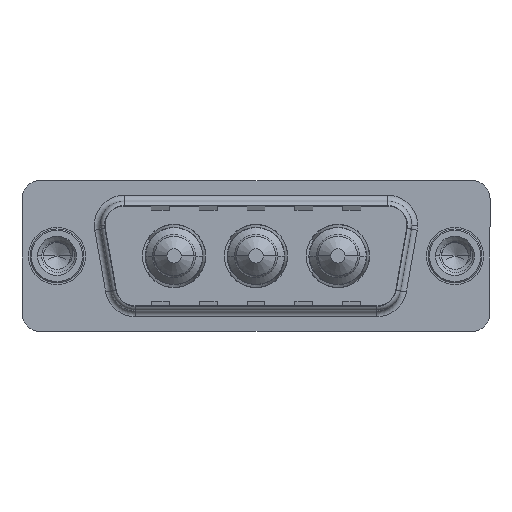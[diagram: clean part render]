
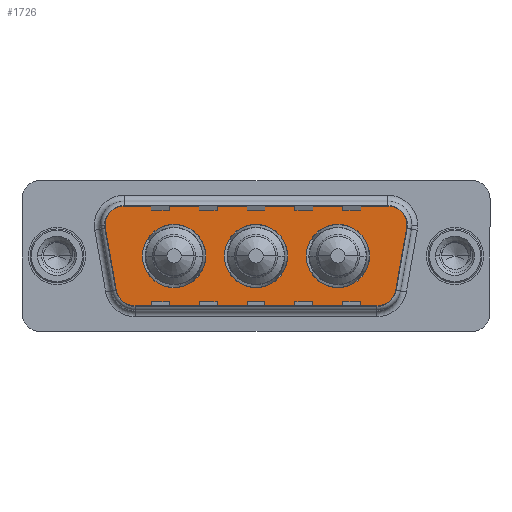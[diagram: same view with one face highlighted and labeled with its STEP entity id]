
A CAD part, top view. The second image highlights one B-rep face of the part: STEP entity #1726.
In plain terms, the highlighted planar face has unit normal (0, 0, 1).
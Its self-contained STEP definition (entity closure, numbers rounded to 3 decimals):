
#42 = DIRECTION ( 'NONE',  ( -1., 0., 0. ) ) ;
#144 = ORIENTED_EDGE ( 'NONE', *, *, #1519, .T. ) ;
#194 = VERTEX_POINT ( 'NONE', #1697 ) ;
#228 = ORIENTED_EDGE ( 'NONE', *, *, #12312, .T. ) ;
#421 = DIRECTION ( 'NONE',  ( 1., 0., 0. ) ) ;
#570 = CIRCLE ( 'NONE', #4856, 2.65 ) ;
#596 = EDGE_CURVE ( 'NONE', #746, #11127, #5800, .T. ) ;
#746 = VERTEX_POINT ( 'NONE', #1865 ) ;
#846 = VERTEX_POINT ( 'NONE', #6445 ) ;
#915 = EDGE_CURVE ( 'NONE', #5797, #9827, #9439, .T. ) ;
#993 = DIRECTION ( 'NONE',  ( 1., 0., 0. ) ) ;
#1413 = AXIS2_PLACEMENT_3D ( 'NONE', #8962, #9779, #2746 ) ;
#1519 = EDGE_CURVE ( 'NONE', #9827, #6201, #9106, .T. ) ;
#1533 = ORIENTED_EDGE ( 'NONE', *, *, #2544, .T. ) ;
#1560 = EDGE_CURVE ( 'NONE', #12996, #7436, #6411, .T. ) ;
#1632 = AXIS2_PLACEMENT_3D ( 'NONE', #11360, #8532, #8520 ) ;
#1697 = CARTESIAN_POINT ( 'NONE',  ( 3.441, 2.553, 0. ) ) ;
#1726 = ADVANCED_FACE ( 'NONE', ( #7830, #2380, #12896, #13206 ), #9777, .T. ) ;
#1814 = DIRECTION ( 'NONE',  ( 0.174, 0.985, 0. ) ) ;
#1865 = CARTESIAN_POINT ( 'NONE',  ( 7.15, 0., 0. ) ) ;
#2040 = VECTOR ( 'NONE', #5356, 1000. ) ;
#2229 = AXIS2_PLACEMENT_3D ( 'NONE', #11794, #5753, #12817 ) ;
#2326 = DIRECTION ( 'NONE',  ( 0., 0., 1. ) ) ;
#2380 = FACE_BOUND ( 'NONE', #3631, .T. ) ;
#2398 = CIRCLE ( 'NONE', #2229, 2.65 ) ;
#2465 = EDGE_CURVE ( 'NONE', #9430, #2941, #10359, .T. ) ;
#2533 = DIRECTION ( 'NONE',  ( -1., 0., 0. ) ) ;
#2544 = EDGE_CURVE ( 'NONE', #194, #12849, #7321, .T. ) ;
#2681 = AXIS2_PLACEMENT_3D ( 'NONE', #4132, #11233, #5159 ) ;
#2745 = ORIENTED_EDGE ( 'NONE', *, *, #2465, .F. ) ;
#2746 = DIRECTION ( 'NONE',  ( 1., 0., 0. ) ) ;
#2854 = ORIENTED_EDGE ( 'NONE', *, *, #5192, .F. ) ;
#2876 = CARTESIAN_POINT ( 'NONE',  ( 6.434, -2.9, 0. ) ) ;
#2888 = CARTESIAN_POINT ( 'NONE',  ( 4.464, -3.247, 0. ) ) ;
#2941 = VERTEX_POINT ( 'NONE', #13060 ) ;
#2987 = ORIENTED_EDGE ( 'NONE', *, *, #1560, .T. ) ;
#3088 = AXIS2_PLACEMENT_3D ( 'NONE', #11510, #12285, #421 ) ;
#3631 = EDGE_LOOP ( 'NONE', ( #2745, #2854 ) ) ;
#3735 = ORIENTED_EDGE ( 'NONE', *, *, #596, .F. ) ;
#3815 = CARTESIAN_POINT ( 'NONE',  ( 5.411, 4.9, 0. ) ) ;
#3872 = LINE ( 'NONE', #3815, #11345 ) ;
#3898 = DIRECTION ( 'NONE',  ( -1., 0., 0. ) ) ;
#3949 = CIRCLE ( 'NONE', #6325, 2. ) ;
#4007 = CARTESIAN_POINT ( 'NONE',  ( 27.889, 2.9, 0. ) ) ;
#4132 = CARTESIAN_POINT ( 'NONE',  ( 9.8, 0., 0. ) ) ;
#4135 = DIRECTION ( 'NONE',  ( 0.174, -0.985, 0. ) ) ;
#4206 = DIRECTION ( 'NONE',  ( 0., 0., 1. ) ) ;
#4333 = VECTOR ( 'NONE', #1814, 1000. ) ;
#4336 = CARTESIAN_POINT ( 'NONE',  ( 6.434, -4.9, 0. ) ) ;
#4523 = ORIENTED_EDGE ( 'NONE', *, *, #8874, .F. ) ;
#4662 = CIRCLE ( 'NONE', #2681, 2.65 ) ;
#4856 = AXIS2_PLACEMENT_3D ( 'NONE', #13230, #7177, #993 ) ;
#4901 = CARTESIAN_POINT ( 'NONE',  ( 26.866, -4.9, 0. ) ) ;
#5159 = DIRECTION ( 'NONE',  ( 1., 0., 0. ) ) ;
#5192 = EDGE_CURVE ( 'NONE', #2941, #9430, #11567, .T. ) ;
#5356 = DIRECTION ( 'NONE',  ( 1., 0., 0. ) ) ;
#5564 = AXIS2_PLACEMENT_3D ( 'NONE', #12219, #6167, #13238 ) ;
#5594 = CARTESIAN_POINT ( 'NONE',  ( 26.866, -2.9, 0. ) ) ;
#5753 = DIRECTION ( 'NONE',  ( 0., 0., 1. ) ) ;
#5797 = VERTEX_POINT ( 'NONE', #4901 ) ;
#5800 = CIRCLE ( 'NONE', #1413, 2.65 ) ;
#5952 = ORIENTED_EDGE ( 'NONE', *, *, #9677, .T. ) ;
#6167 = DIRECTION ( 'NONE',  ( 0., 0., 1. ) ) ;
#6201 = VERTEX_POINT ( 'NONE', #11793 ) ;
#6240 = DIRECTION ( 'NONE',  ( 0., 0., 1. ) ) ;
#6325 = AXIS2_PLACEMENT_3D ( 'NONE', #2876, #10010, #3898 ) ;
#6411 = CIRCLE ( 'NONE', #9571, 2. ) ;
#6445 = CARTESIAN_POINT ( 'NONE',  ( 6.434, -4.9, 0. ) ) ;
#6612 = CARTESIAN_POINT ( 'NONE',  ( 28.836, -3.247, 0. ) ) ;
#6669 = EDGE_LOOP ( 'NONE', ( #7057, #144, #9351, #2987, #9193, #228, #1533, #11855, #5952 ) ) ;
#6882 = CARTESIAN_POINT ( 'NONE',  ( 29.859, 2.553, 0. ) ) ;
#6904 = ORIENTED_EDGE ( 'NONE', *, *, #8582, .F. ) ;
#7029 = VECTOR ( 'NONE', #4135, 1000. ) ;
#7057 = ORIENTED_EDGE ( 'NONE', *, *, #915, .T. ) ;
#7070 = CARTESIAN_POINT ( 'NONE',  ( 26.15, 0., 0. ) ) ;
#7177 = DIRECTION ( 'NONE',  ( 0., 0., 1. ) ) ;
#7321 = LINE ( 'NONE', #12306, #7029 ) ;
#7436 = VERTEX_POINT ( 'NONE', #9846 ) ;
#7498 = LINE ( 'NONE', #4336, #2040 ) ;
#7830 = FACE_BOUND ( 'NONE', #8534, .T. ) ;
#8129 = EDGE_CURVE ( 'NONE', #7436, #9442, #3872, .T. ) ;
#8520 = DIRECTION ( 'NONE',  ( 1., 0., 0. ) ) ;
#8531 = CIRCLE ( 'NONE', #5564, 2. ) ;
#8532 = DIRECTION ( 'NONE',  ( 0., 0., 1. ) ) ;
#8534 = EDGE_LOOP ( 'NONE', ( #10165, #6904 ) ) ;
#8582 = EDGE_CURVE ( 'NONE', #12818, #11789, #2398, .T. ) ;
#8832 = DIRECTION ( 'NONE',  ( 1., 0., 0. ) ) ;
#8874 = EDGE_CURVE ( 'NONE', #11127, #746, #4662, .T. ) ;
#8962 = CARTESIAN_POINT ( 'NONE',  ( 9.8, 0., 0. ) ) ;
#9106 = LINE ( 'NONE', #6882, #4333 ) ;
#9193 = ORIENTED_EDGE ( 'NONE', *, *, #8129, .T. ) ;
#9320 = CARTESIAN_POINT ( 'NONE',  ( 19.3, 0., 0. ) ) ;
#9351 = ORIENTED_EDGE ( 'NONE', *, *, #13010, .T. ) ;
#9430 = VERTEX_POINT ( 'NONE', #7070 ) ;
#9439 = CIRCLE ( 'NONE', #12097, 2. ) ;
#9442 = VERTEX_POINT ( 'NONE', #11130 ) ;
#9571 = AXIS2_PLACEMENT_3D ( 'NONE', #4007, #4206, #2533 ) ;
#9677 = EDGE_CURVE ( 'NONE', #846, #5797, #7498, .T. ) ;
#9777 = PLANE ( 'NONE',  #10007 ) ;
#9779 = DIRECTION ( 'NONE',  ( 0., 0., 1. ) ) ;
#9827 = VERTEX_POINT ( 'NONE', #6612 ) ;
#9846 = CARTESIAN_POINT ( 'NONE',  ( 27.889, 4.9, 0. ) ) ;
#9929 = DIRECTION ( 'NONE',  ( -1., 0., 0. ) ) ;
#10007 = AXIS2_PLACEMENT_3D ( 'NONE', #5594, #2326, #12087 ) ;
#10010 = DIRECTION ( 'NONE',  ( 0., 0., 1. ) ) ;
#10092 = EDGE_CURVE ( 'NONE', #11789, #12818, #570, .T. ) ;
#10165 = ORIENTED_EDGE ( 'NONE', *, *, #10092, .F. ) ;
#10359 = CIRCLE ( 'NONE', #3088, 2.65 ) ;
#10669 = EDGE_LOOP ( 'NONE', ( #4523, #3735 ) ) ;
#10964 = CARTESIAN_POINT ( 'NONE',  ( 12.45, 0., 0. ) ) ;
#11030 = CARTESIAN_POINT ( 'NONE',  ( 26.866, -2.9, 0. ) ) ;
#11119 = DIRECTION ( 'NONE',  ( 0., 0., 1. ) ) ;
#11127 = VERTEX_POINT ( 'NONE', #10964 ) ;
#11130 = CARTESIAN_POINT ( 'NONE',  ( 5.411, 4.9, 0. ) ) ;
#11233 = DIRECTION ( 'NONE',  ( 0., 0., 1. ) ) ;
#11240 = CARTESIAN_POINT ( 'NONE',  ( 29.889, 2.9, 0. ) ) ;
#11345 = VECTOR ( 'NONE', #9929, 1000. ) ;
#11360 = CARTESIAN_POINT ( 'NONE',  ( 23.5, 0., 0. ) ) ;
#11510 = CARTESIAN_POINT ( 'NONE',  ( 23.5, 0., 0. ) ) ;
#11539 = EDGE_CURVE ( 'NONE', #12849, #846, #3949, .T. ) ;
#11567 = CIRCLE ( 'NONE', #1632, 2.65 ) ;
#11789 = VERTEX_POINT ( 'NONE', #9320 ) ;
#11793 = CARTESIAN_POINT ( 'NONE',  ( 29.859, 2.553, 0. ) ) ;
#11794 = CARTESIAN_POINT ( 'NONE',  ( 16.65, 0., 0. ) ) ;
#11855 = ORIENTED_EDGE ( 'NONE', *, *, #11539, .T. ) ;
#11940 = CARTESIAN_POINT ( 'NONE',  ( 14., 0., 0. ) ) ;
#12001 = CIRCLE ( 'NONE', #12575, 2. ) ;
#12087 = DIRECTION ( 'NONE',  ( 1., 0., 0. ) ) ;
#12097 = AXIS2_PLACEMENT_3D ( 'NONE', #11030, #11119, #8832 ) ;
#12219 = CARTESIAN_POINT ( 'NONE',  ( 5.411, 2.9, 0. ) ) ;
#12285 = DIRECTION ( 'NONE',  ( 0., 0., 1. ) ) ;
#12287 = CARTESIAN_POINT ( 'NONE',  ( 27.889, 2.9, 0. ) ) ;
#12306 = CARTESIAN_POINT ( 'NONE',  ( 3.441, 2.553, 0. ) ) ;
#12312 = EDGE_CURVE ( 'NONE', #9442, #194, #8531, .T. ) ;
#12575 = AXIS2_PLACEMENT_3D ( 'NONE', #12287, #6240, #42 ) ;
#12817 = DIRECTION ( 'NONE',  ( 1., 0., 0. ) ) ;
#12818 = VERTEX_POINT ( 'NONE', #11940 ) ;
#12849 = VERTEX_POINT ( 'NONE', #2888 ) ;
#12896 = FACE_BOUND ( 'NONE', #10669, .T. ) ;
#12996 = VERTEX_POINT ( 'NONE', #11240 ) ;
#13010 = EDGE_CURVE ( 'NONE', #6201, #12996, #12001, .T. ) ;
#13060 = CARTESIAN_POINT ( 'NONE',  ( 20.85, 0., 0. ) ) ;
#13206 = FACE_OUTER_BOUND ( 'NONE', #6669, .T. ) ;
#13230 = CARTESIAN_POINT ( 'NONE',  ( 16.65, 0., 0. ) ) ;
#13238 = DIRECTION ( 'NONE',  ( 1., 0., 0. ) ) ;
